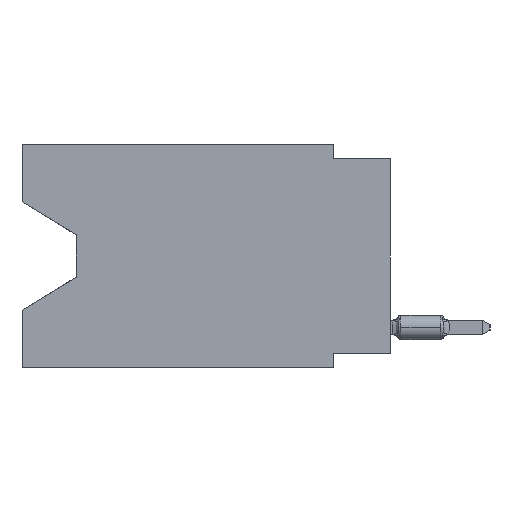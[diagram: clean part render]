
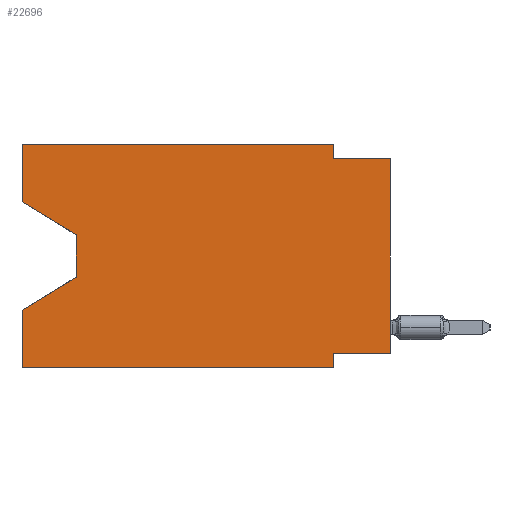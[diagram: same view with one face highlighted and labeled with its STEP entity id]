
A CAD part, left-side view. The second image highlights one B-rep face of the part: STEP entity #22696.
In plain terms, the highlighted planar face has unit normal (-1, 0, 0).
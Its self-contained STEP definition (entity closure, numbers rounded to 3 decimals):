
#23 = EDGE_CURVE ( 'NONE', #37033, #45108, #23939, .T. ) ;
#550 = DIRECTION ( 'NONE',  ( 0., 0., 1. ) ) ;
#1431 = CARTESIAN_POINT ( 'NONE',  ( 0., 16.383, 0. ) ) ;
#1752 = DIRECTION ( 'NONE',  ( 0., 0., 1. ) ) ;
#1789 = VERTEX_POINT ( 'NONE', #26051 ) ;
#2447 = CARTESIAN_POINT ( 'NONE',  ( 0., 0., -9.271 ) ) ;
#2922 = EDGE_CURVE ( 'NONE', #15304, #37033, #29207, .T. ) ;
#3065 = ORIENTED_EDGE ( 'NONE', *, *, #23, .F. ) ;
#3474 = VERTEX_POINT ( 'NONE', #45961 ) ;
#3957 = ORIENTED_EDGE ( 'NONE', *, *, #54836, .F. ) ;
#4242 = CARTESIAN_POINT ( 'NONE',  ( 0., 13.97, -4.013 ) ) ;
#4258 = EDGE_CURVE ( 'NONE', #15582, #1789, #54494, .T. ) ;
#4500 = CARTESIAN_POINT ( 'NONE',  ( 0., 2.54, 0. ) ) ;
#5266 = ORIENTED_EDGE ( 'NONE', *, *, #39689, .T. ) ;
#6011 = DIRECTION ( 'NONE',  ( 0., -1., 0. ) ) ;
#6442 = ORIENTED_EDGE ( 'NONE', *, *, #41197, .T. ) ;
#7035 = CARTESIAN_POINT ( 'NONE',  ( 0., 13.97, -5.893 ) ) ;
#10746 = ORIENTED_EDGE ( 'NONE', *, *, #19393, .F. ) ;
#12031 = VECTOR ( 'NONE', #15833, 1000. ) ;
#12962 = CARTESIAN_POINT ( 'NONE',  ( 0., 13.97, -4.013 ) ) ;
#13684 = CARTESIAN_POINT ( 'NONE',  ( 0., 2.54, -9.271 ) ) ;
#14261 = DIRECTION ( 'NONE',  ( 0., 0., -1. ) ) ;
#15304 = VERTEX_POINT ( 'NONE', #38786 ) ;
#15546 = CARTESIAN_POINT ( 'NONE',  ( 0., 16.383, -9.906 ) ) ;
#15582 = VERTEX_POINT ( 'NONE', #30506 ) ;
#15833 = DIRECTION ( 'NONE',  ( 0., 0.855, -0.519 ) ) ;
#15949 = LINE ( 'NONE', #2447, #56525 ) ;
#16493 = VERTEX_POINT ( 'NONE', #12962 ) ;
#18137 = DIRECTION ( 'NONE',  ( 1., 0., 0. ) ) ;
#18441 = VECTOR ( 'NONE', #30643, 1000. ) ;
#18860 = VECTOR ( 'NONE', #6011, 1000. ) ;
#19086 = CARTESIAN_POINT ( 'NONE',  ( 0., 2.54, 0. ) ) ;
#19393 = EDGE_CURVE ( 'NONE', #24281, #47127, #15949, .T. ) ;
#19598 = EDGE_CURVE ( 'NONE', #3474, #23315, #34385, .T. ) ;
#20341 = LINE ( 'NONE', #38885, #32271 ) ;
#21017 = VERTEX_POINT ( 'NONE', #23849 ) ;
#21791 = EDGE_LOOP ( 'NONE', ( #54144, #6442, #22092, #45677, #5266, #62125, #10746, #43162, #54087, #3957, #3065, #41357 ) ) ;
#22092 = ORIENTED_EDGE ( 'NONE', *, *, #4258, .T. ) ;
#22696 = ADVANCED_FACE ( 'NONE', ( #51448 ), #46734, .F. ) ;
#22851 = VECTOR ( 'NONE', #53279, 1000. ) ;
#22870 = DIRECTION ( 'NONE',  ( 0., 0., -1. ) ) ;
#22903 = LINE ( 'NONE', #19086, #39257 ) ;
#23315 = VERTEX_POINT ( 'NONE', #61229 ) ;
#23849 = CARTESIAN_POINT ( 'NONE',  ( 0., 2.54, -9.906 ) ) ;
#23939 = LINE ( 'NONE', #38405, #18860 ) ;
#24281 = VERTEX_POINT ( 'NONE', #34666 ) ;
#25319 = CARTESIAN_POINT ( 'NONE',  ( 0., 2.54, -9.906 ) ) ;
#26051 = CARTESIAN_POINT ( 'NONE',  ( 0., 16.383, -7.36 ) ) ;
#28977 = VECTOR ( 'NONE', #56500, 1000. ) ;
#29207 = LINE ( 'NONE', #30370, #44024 ) ;
#29969 = DIRECTION ( 'NONE',  ( 0., -1., 0. ) ) ;
#30278 = CARTESIAN_POINT ( 'NONE',  ( 0., 0., -0.635 ) ) ;
#30370 = CARTESIAN_POINT ( 'NONE',  ( 0., 16.383, 0. ) ) ;
#30434 = DIRECTION ( 'NONE',  ( 0., 1., 0. ) ) ;
#30506 = CARTESIAN_POINT ( 'NONE',  ( 0., 13.97, -5.893 ) ) ;
#30643 = DIRECTION ( 'NONE',  ( 0., 0., -1. ) ) ;
#32271 = VECTOR ( 'NONE', #550, 1000. ) ;
#33746 = EDGE_CURVE ( 'NONE', #61771, #1789, #61501, .T. ) ;
#34385 = LINE ( 'NONE', #30278, #50350 ) ;
#34666 = CARTESIAN_POINT ( 'NONE',  ( 0., 0., -9.271 ) ) ;
#34739 = CARTESIAN_POINT ( 'NONE',  ( 0., 16.383, -9.906 ) ) ;
#36998 = VECTOR ( 'NONE', #45240, 1000. ) ;
#37033 = VERTEX_POINT ( 'NONE', #1431 ) ;
#38405 = CARTESIAN_POINT ( 'NONE',  ( 0., 16.383, 0. ) ) ;
#38786 = CARTESIAN_POINT ( 'NONE',  ( 0., 16.383, -2.546 ) ) ;
#38885 = CARTESIAN_POINT ( 'NONE',  ( 0., 0., 0. ) ) ;
#39257 = VECTOR ( 'NONE', #46462, 1000. ) ;
#39689 = EDGE_CURVE ( 'NONE', #61771, #21017, #58905, .T. ) ;
#41197 = EDGE_CURVE ( 'NONE', #16493, #15582, #61092, .T. ) ;
#41357 = ORIENTED_EDGE ( 'NONE', *, *, #2922, .F. ) ;
#43162 = ORIENTED_EDGE ( 'NONE', *, *, #54874, .T. ) ;
#44024 = VECTOR ( 'NONE', #1752, 1000. ) ;
#44153 = LINE ( 'NONE', #25319, #18441 ) ;
#45108 = VERTEX_POINT ( 'NONE', #4500 ) ;
#45240 = DIRECTION ( 'NONE',  ( 0., -0.855, -0.519 ) ) ;
#45677 = ORIENTED_EDGE ( 'NONE', *, *, #33746, .F. ) ;
#45961 = CARTESIAN_POINT ( 'NONE',  ( 0., 2.54, -0.635 ) ) ;
#46105 = CARTESIAN_POINT ( 'NONE',  ( 0., 16.383, 0. ) ) ;
#46462 = DIRECTION ( 'NONE',  ( 0., 0., -1. ) ) ;
#46734 = PLANE ( 'NONE',  #50575 ) ;
#47127 = VERTEX_POINT ( 'NONE', #13684 ) ;
#49941 = CARTESIAN_POINT ( 'NONE',  ( 0., 16.383, -2.546 ) ) ;
#50350 = VECTOR ( 'NONE', #29969, 1000. ) ;
#50575 = AXIS2_PLACEMENT_3D ( 'NONE', #46105, #18137, #22870 ) ;
#51448 = FACE_OUTER_BOUND ( 'NONE', #21791, .T. ) ;
#53257 = VECTOR ( 'NONE', #14261, 1000. ) ;
#53279 = DIRECTION ( 'NONE',  ( 0., -1., 0. ) ) ;
#53796 = EDGE_CURVE ( 'NONE', #15304, #16493, #55294, .T. ) ;
#54087 = ORIENTED_EDGE ( 'NONE', *, *, #19598, .F. ) ;
#54144 = ORIENTED_EDGE ( 'NONE', *, *, #53796, .T. ) ;
#54494 = LINE ( 'NONE', #7035, #12031 ) ;
#54836 = EDGE_CURVE ( 'NONE', #45108, #3474, #22903, .T. ) ;
#54874 = EDGE_CURVE ( 'NONE', #24281, #23315, #20341, .T. ) ;
#55294 = LINE ( 'NONE', #49941, #36998 ) ;
#56500 = DIRECTION ( 'NONE',  ( 0., 0., 1. ) ) ;
#56525 = VECTOR ( 'NONE', #30434, 1000. ) ;
#58905 = LINE ( 'NONE', #34739, #22851 ) ;
#59002 = EDGE_CURVE ( 'NONE', #47127, #21017, #44153, .T. ) ;
#61092 = LINE ( 'NONE', #4242, #53257 ) ;
#61229 = CARTESIAN_POINT ( 'NONE',  ( 0., 0., -0.635 ) ) ;
#61501 = LINE ( 'NONE', #62101, #28977 ) ;
#61771 = VERTEX_POINT ( 'NONE', #15546 ) ;
#62101 = CARTESIAN_POINT ( 'NONE',  ( 0., 16.383, 0. ) ) ;
#62125 = ORIENTED_EDGE ( 'NONE', *, *, #59002, .F. ) ;
